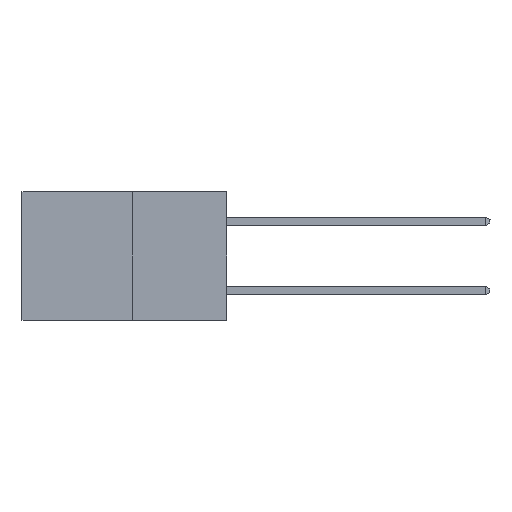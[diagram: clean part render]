
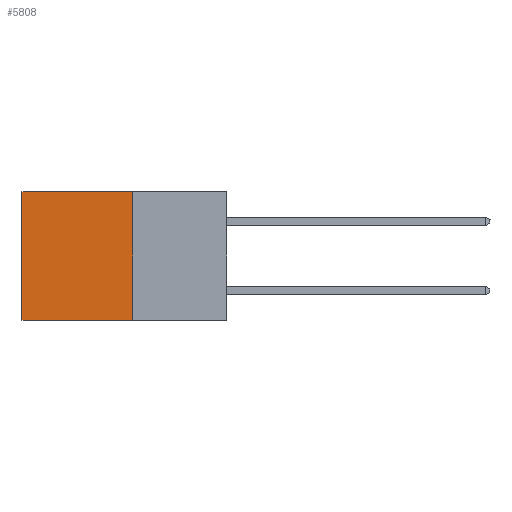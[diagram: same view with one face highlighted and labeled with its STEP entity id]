
A CAD part, left-side view. The second image highlights one B-rep face of the part: STEP entity #5808.
In plain terms, the highlighted planar face has unit normal (-1, 0, 0).
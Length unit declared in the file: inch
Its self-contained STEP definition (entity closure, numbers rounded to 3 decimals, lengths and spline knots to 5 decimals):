
#16 = VERTEX_POINT ( 'NONE', #8754 ) ;
#432 = LINE ( 'NONE', #3126, #2763 ) ;
#733 = FACE_OUTER_BOUND ( 'NONE', #6558, .T. ) ;
#778 = VERTEX_POINT ( 'NONE', #5669 ) ;
#974 = ORIENTED_EDGE ( 'NONE', *, *, #2576, .F. ) ;
#1224 = EDGE_CURVE ( 'NONE', #778, #6737, #432, .T. ) ;
#1855 = CARTESIAN_POINT ( 'NONE',  ( 0.277, 0.59, -0.37 ) ) ;
#2115 = DIRECTION ( 'NONE',  ( 0., 0., -1. ) ) ;
#2576 = EDGE_CURVE ( 'NONE', #9288, #778, #2867, .T. ) ;
#2763 = VECTOR ( 'NONE', #6455, 39.37008 ) ;
#2867 = LINE ( 'NONE', #7632, #5057 ) ;
#2910 = VECTOR ( 'NONE', #2115, 39.37008 ) ;
#3126 = CARTESIAN_POINT ( 'NONE',  ( 0.277, 0.27, -0.37 ) ) ;
#3130 = AXIS2_PLACEMENT_3D ( 'NONE', #3552, #3464, #3455 ) ;
#3277 = ORIENTED_EDGE ( 'NONE', *, *, #9709, .T. ) ;
#3455 = DIRECTION ( 'NONE',  ( 0., 0., -1. ) ) ;
#3464 = DIRECTION ( 'NONE',  ( 1., 0., 0. ) ) ;
#3476 = PLANE ( 'NONE',  #3130 ) ;
#3552 = CARTESIAN_POINT ( 'NONE',  ( 0.277, 0.27, -0.37 ) ) ;
#5057 = VECTOR ( 'NONE', #9766, 39.37008 ) ;
#5195 = ORIENTED_EDGE ( 'NONE', *, *, #6107, .T. ) ;
#5669 = CARTESIAN_POINT ( 'NONE',  ( 0.277, 0.27, -0.37 ) ) ;
#5808 = ADVANCED_FACE ( 'NONE', ( #733 ), #3476, .F. ) ;
#6047 = CARTESIAN_POINT ( 'NONE',  ( 0.277, 0.27, 0. ) ) ;
#6107 = EDGE_CURVE ( 'NONE', #16, #6737, #7258, .T. ) ;
#6455 = DIRECTION ( 'NONE',  ( 0., 1., 0. ) ) ;
#6558 = EDGE_LOOP ( 'NONE', ( #5195, #7358, #974, #3277 ) ) ;
#6737 = VERTEX_POINT ( 'NONE', #9604 ) ;
#7093 = LINE ( 'NONE', #9828, #8968 ) ;
#7258 = LINE ( 'NONE', #1855, #2910 ) ;
#7358 = ORIENTED_EDGE ( 'NONE', *, *, #1224, .F. ) ;
#7632 = CARTESIAN_POINT ( 'NONE',  ( 0.277, 0.27, -0.37 ) ) ;
#8279 = DIRECTION ( 'NONE',  ( 0., 1., 0. ) ) ;
#8754 = CARTESIAN_POINT ( 'NONE',  ( 0.277, 0.59, 0. ) ) ;
#8968 = VECTOR ( 'NONE', #8279, 39.37008 ) ;
#9288 = VERTEX_POINT ( 'NONE', #6047 ) ;
#9604 = CARTESIAN_POINT ( 'NONE',  ( 0.277, 0.59, -0.37 ) ) ;
#9709 = EDGE_CURVE ( 'NONE', #9288, #16, #7093, .T. ) ;
#9766 = DIRECTION ( 'NONE',  ( 0., 0., -1. ) ) ;
#9828 = CARTESIAN_POINT ( 'NONE',  ( 0.277, 0.27, 0. ) ) ;
